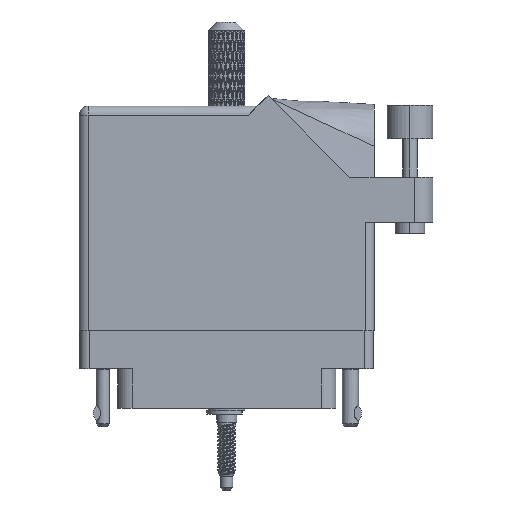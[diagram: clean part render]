
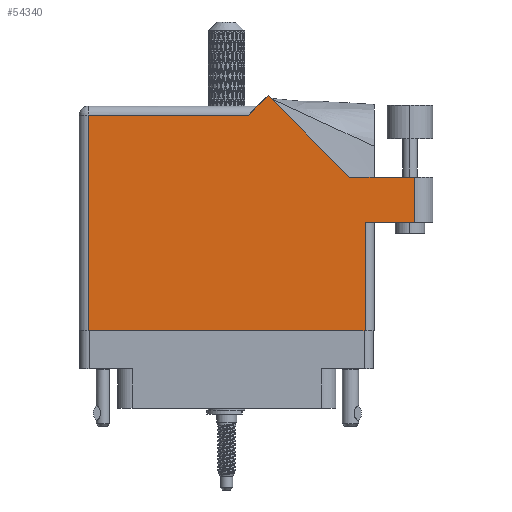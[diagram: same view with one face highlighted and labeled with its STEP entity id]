
A CAD part, front view. The second image highlights one B-rep face of the part: STEP entity #54340.
In plain terms, the highlighted face is planar.
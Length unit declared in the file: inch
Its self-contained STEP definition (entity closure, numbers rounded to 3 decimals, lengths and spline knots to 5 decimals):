
#3718 = DIRECTION ( 'NONE',  ( 0., 1., 0. ) ) ;
#3758 = ORIENTED_EDGE ( 'NONE', *, *, #54750, .T. ) ;
#4078 = CARTESIAN_POINT ( 'NONE',  ( 1.948, 0.737, 0. ) ) ;
#4619 = CARTESIAN_POINT ( 'NONE',  ( 2.285, 0.737, 0. ) ) ;
#7697 = ORIENTED_EDGE ( 'NONE', *, *, #111378, .T. ) ;
#10456 = DIRECTION ( 'NONE',  ( 0., 1., 0. ) ) ;
#12656 = CARTESIAN_POINT ( 'NONE',  ( 0.062, 1.468, 0. ) ) ;
#12945 = CARTESIAN_POINT ( 'NONE',  ( 1.948, 0.737, 0. ) ) ;
#16075 = CARTESIAN_POINT ( 'NONE',  ( 2.01, 0.737, 0. ) ) ;
#16412 = ORIENTED_EDGE ( 'NONE', *, *, #97557, .T. ) ;
#17344 = FACE_OUTER_BOUND ( 'NONE', #22899, .T. ) ;
#18868 = CARTESIAN_POINT ( 'NONE',  ( 1.84442, 1.044, 0. ) ) ;
#19280 = CARTESIAN_POINT ( 'NONE',  ( 2.285, 1.044, 0. ) ) ;
#19556 = LINE ( 'NONE', #39850, #110253 ) ;
#20492 = EDGE_CURVE ( 'NONE', #46188, #41649, #103647, .T. ) ;
#21169 = ORIENTED_EDGE ( 'NONE', *, *, #113765, .T. ) ;
#22899 = EDGE_LOOP ( 'NONE', ( #3758, #21169, #54110, #16412, #104142, #88917, #7697, #87473, #82892 ) ) ;
#24796 = CARTESIAN_POINT ( 'NONE',  ( 1.948, 0., 0. ) ) ;
#30794 = VECTOR ( 'NONE', #33350, 39.37008 ) ;
#31093 = VECTOR ( 'NONE', #93827, 39.37008 ) ;
#32969 = CARTESIAN_POINT ( 'NONE',  ( 0.062, 0., 0. ) ) ;
#33211 = VERTEX_POINT ( 'NONE', #12945 ) ;
#33350 = DIRECTION ( 'NONE',  ( 1., 0., 0. ) ) ;
#34892 = CARTESIAN_POINT ( 'NONE',  ( 0., 0., 0. ) ) ;
#37610 = LINE ( 'NONE', #49771, #53987 ) ;
#37891 = LINE ( 'NONE', #19280, #72228 ) ;
#37995 = CARTESIAN_POINT ( 'NONE',  ( 2.285, 1.044, 0. ) ) ;
#39850 = CARTESIAN_POINT ( 'NONE',  ( 0., 1.468, 0. ) ) ;
#41649 = VERTEX_POINT ( 'NONE', #94804 ) ;
#45309 = VECTOR ( 'NONE', #70478, 39.37008 ) ;
#46188 = VERTEX_POINT ( 'NONE', #102527 ) ;
#49088 = DIRECTION ( 'NONE',  ( -1., 0., 0. ) ) ;
#49771 = CARTESIAN_POINT ( 'NONE',  ( 1.84442, 1.044, 0. ) ) ;
#50408 = CARTESIAN_POINT ( 'NONE',  ( 2.41, 1.044, 0. ) ) ;
#50515 = VERTEX_POINT ( 'NONE', #37995 ) ;
#52507 = EDGE_CURVE ( 'NONE', #112731, #33211, #98645, .T. ) ;
#53139 = DIRECTION ( 'NONE',  ( -1., 0., 0. ) ) ;
#53987 = VECTOR ( 'NONE', #94307, 39.37008 ) ;
#54110 = ORIENTED_EDGE ( 'NONE', *, *, #102965, .T. ) ;
#54340 = ADVANCED_FACE ( 'NONE', ( #17344 ), #96967, .F. ) ;
#54750 = EDGE_CURVE ( 'NONE', #33211, #72992, #55852, .T. ) ;
#55777 = DIRECTION ( 'NONE',  ( -0.707, -0.707, 0. ) ) ;
#55852 = LINE ( 'NONE', #16075, #81991 ) ;
#60184 = AXIS2_PLACEMENT_3D ( 'NONE', #61984, #97686, #53139 ) ;
#61984 = CARTESIAN_POINT ( 'NONE',  ( 0., 1.53, 0. ) ) ;
#62432 = LINE ( 'NONE', #34892, #30794 ) ;
#66473 = VECTOR ( 'NONE', #55777, 39.37008 ) ;
#67899 = DIRECTION ( 'NONE',  ( 1., 0., 0. ) ) ;
#70478 = DIRECTION ( 'NONE',  ( 0., -1., 0. ) ) ;
#71158 = VECTOR ( 'NONE', #3718, 39.37008 ) ;
#71330 = EDGE_CURVE ( 'NONE', #41649, #83704, #19556, .T. ) ;
#72228 = VECTOR ( 'NONE', #10456, 39.37008 ) ;
#72992 = VERTEX_POINT ( 'NONE', #4619 ) ;
#73448 = CARTESIAN_POINT ( 'NONE',  ( 1.217, 1.53, 0. ) ) ;
#78171 = CARTESIAN_POINT ( 'NONE',  ( 0.062, 0., 0. ) ) ;
#79966 = VERTEX_POINT ( 'NONE', #32969 ) ;
#81039 = LINE ( 'NONE', #78171, #45309 ) ;
#81991 = VECTOR ( 'NONE', #67899, 39.37008 ) ;
#82892 = ORIENTED_EDGE ( 'NONE', *, *, #52507, .T. ) ;
#83704 = VERTEX_POINT ( 'NONE', #12656 ) ;
#83964 = EDGE_CURVE ( 'NONE', #79966, #112731, #62432, .T. ) ;
#87473 = ORIENTED_EDGE ( 'NONE', *, *, #83964, .T. ) ;
#88917 = ORIENTED_EDGE ( 'NONE', *, *, #71330, .T. ) ;
#93827 = DIRECTION ( 'NONE',  ( -1., 0., 0. ) ) ;
#94307 = DIRECTION ( 'NONE',  ( -0.707, 0.707, 0. ) ) ;
#94804 = CARTESIAN_POINT ( 'NONE',  ( 1.155, 1.468, 0. ) ) ;
#96967 = PLANE ( 'NONE',  #60184 ) ;
#97557 = EDGE_CURVE ( 'NONE', #108785, #46188, #37610, .T. ) ;
#97686 = DIRECTION ( 'NONE',  ( 0., 0., -1. ) ) ;
#98645 = LINE ( 'NONE', #4078, #71158 ) ;
#102527 = CARTESIAN_POINT ( 'NONE',  ( 1.28771, 1.60071, 0. ) ) ;
#102965 = EDGE_CURVE ( 'NONE', #50515, #108785, #108026, .T. ) ;
#103647 = LINE ( 'NONE', #73448, #66473 ) ;
#104142 = ORIENTED_EDGE ( 'NONE', *, *, #20492, .T. ) ;
#108026 = LINE ( 'NONE', #50408, #31093 ) ;
#108785 = VERTEX_POINT ( 'NONE', #18868 ) ;
#110253 = VECTOR ( 'NONE', #49088, 39.37008 ) ;
#111378 = EDGE_CURVE ( 'NONE', #83704, #79966, #81039, .T. ) ;
#112731 = VERTEX_POINT ( 'NONE', #24796 ) ;
#113765 = EDGE_CURVE ( 'NONE', #72992, #50515, #37891, .T. ) ;
